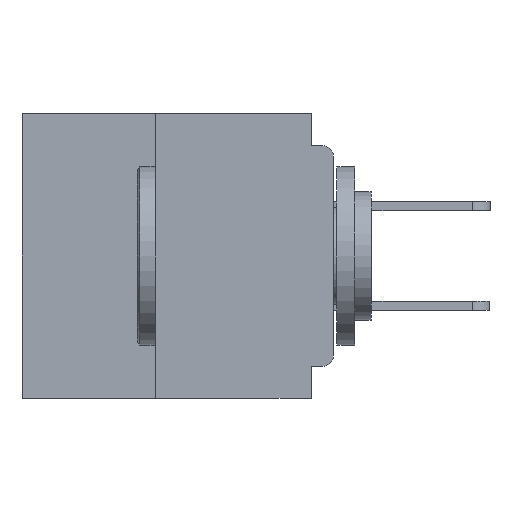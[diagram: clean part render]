
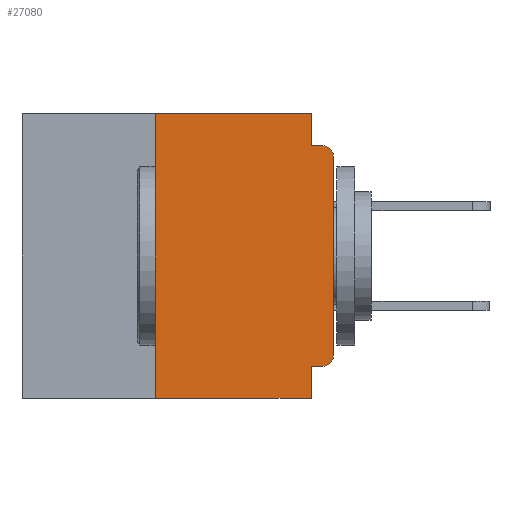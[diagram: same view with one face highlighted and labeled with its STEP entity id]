
A CAD part, left-side view. The second image highlights one B-rep face of the part: STEP entity #27080.
In plain terms, the highlighted planar face has unit normal (-1, 0, 0).
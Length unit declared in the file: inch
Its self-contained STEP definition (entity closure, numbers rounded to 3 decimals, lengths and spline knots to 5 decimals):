
#109 = EDGE_CURVE ( 'NONE', #25057, #23558, #26745, .T. ) ;
#2003 = CARTESIAN_POINT ( 'NONE',  ( 0., 0., -0.355 ) ) ;
#2442 = VERTEX_POINT ( 'NONE', #8196 ) ;
#2882 = DIRECTION ( 'NONE',  ( 0., 0., -1. ) ) ;
#3106 = LINE ( 'NONE', #30872, #19224 ) ;
#3540 = LINE ( 'NONE', #25709, #32822 ) ;
#3785 = CARTESIAN_POINT ( 'NONE',  ( 0., 0.031, 0. ) ) ;
#4992 = DIRECTION ( 'NONE',  ( 0., 1., 0. ) ) ;
#5091 = AXIS2_PLACEMENT_3D ( 'NONE', #8103, #27973, #10960 ) ;
#5327 = DIRECTION ( 'NONE',  ( 0., 0., 1. ) ) ;
#6253 = DIRECTION ( 'NONE',  ( 0., -1., 0. ) ) ;
#6867 = CARTESIAN_POINT ( 'NONE',  ( 0., 0.437, -0.4 ) ) ;
#7379 = DIRECTION ( 'NONE',  ( 0., -1., 0. ) ) ;
#8103 = CARTESIAN_POINT ( 'NONE',  ( 0., 0.015, -0.06 ) ) ;
#8196 = CARTESIAN_POINT ( 'NONE',  ( 0., 0., -0.34 ) ) ;
#8648 = CARTESIAN_POINT ( 'NONE',  ( 0., 0.25, 0. ) ) ;
#8846 = DIRECTION ( 'NONE',  ( -1., 0., 0. ) ) ;
#9642 = VERTEX_POINT ( 'NONE', #13099 ) ;
#9907 = VERTEX_POINT ( 'NONE', #28285 ) ;
#10299 = CARTESIAN_POINT ( 'NONE',  ( 0., 0.015, -0.045 ) ) ;
#10960 = DIRECTION ( 'NONE',  ( 0., 0., -1. ) ) ;
#11476 = VERTEX_POINT ( 'NONE', #10299 ) ;
#12678 = CARTESIAN_POINT ( 'NONE',  ( 0., 0.437, 0. ) ) ;
#13099 = CARTESIAN_POINT ( 'NONE',  ( 0., 0.031, -0.355 ) ) ;
#13114 = EDGE_LOOP ( 'NONE', ( #16177, #21460, #27855, #14474, #21971, #17206, #25708, #18022, #17857, #15685 ) ) ;
#13193 = EDGE_CURVE ( 'NONE', #27193, #2442, #21022, .T. ) ;
#13708 = EDGE_CURVE ( 'NONE', #25057, #18121, #3106, .T. ) ;
#13821 = EDGE_CURVE ( 'NONE', #9642, #23558, #36325, .T. ) ;
#14393 = LINE ( 'NONE', #2003, #35874 ) ;
#14474 = ORIENTED_EDGE ( 'NONE', *, *, #21185, .F. ) ;
#14938 = VECTOR ( 'NONE', #15388, 39.37008 ) ;
#15388 = DIRECTION ( 'NONE',  ( 0., 0., -1. ) ) ;
#15480 = LINE ( 'NONE', #35426, #22037 ) ;
#15609 = DIRECTION ( 'NONE',  ( 0., 0., -1. ) ) ;
#15685 = ORIENTED_EDGE ( 'NONE', *, *, #13193, .T. ) ;
#15722 = VECTOR ( 'NONE', #2882, 39.37008 ) ;
#16177 = ORIENTED_EDGE ( 'NONE', *, *, #30389, .T. ) ;
#16541 = CARTESIAN_POINT ( 'NONE',  ( 0., 0.031, -0.4 ) ) ;
#16759 = CIRCLE ( 'NONE', #5091, 0.015 ) ;
#17206 = ORIENTED_EDGE ( 'NONE', *, *, #13708, .F. ) ;
#17857 = ORIENTED_EDGE ( 'NONE', *, *, #22279, .F. ) ;
#18022 = ORIENTED_EDGE ( 'NONE', *, *, #13821, .F. ) ;
#18121 = VERTEX_POINT ( 'NONE', #8648 ) ;
#19160 = EDGE_CURVE ( 'NONE', #18121, #25252, #3540, .T. ) ;
#19224 = VECTOR ( 'NONE', #5327, 39.37008 ) ;
#19228 = VECTOR ( 'NONE', #6253, 39.37008 ) ;
#19791 = VERTEX_POINT ( 'NONE', #25541 ) ;
#21022 = CIRCLE ( 'NONE', #32841, 0.015 ) ;
#21185 = EDGE_CURVE ( 'NONE', #25252, #19791, #29005, .T. ) ;
#21460 = ORIENTED_EDGE ( 'NONE', *, *, #32525, .T. ) ;
#21971 = ORIENTED_EDGE ( 'NONE', *, *, #19160, .F. ) ;
#22037 = VECTOR ( 'NONE', #7379, 39.37008 ) ;
#22279 = EDGE_CURVE ( 'NONE', #27193, #9642, #14393, .T. ) ;
#22862 = CARTESIAN_POINT ( 'NONE',  ( 0., 0.031, -0.4 ) ) ;
#23393 = CARTESIAN_POINT ( 'NONE',  ( 0., 0., 0. ) ) ;
#23558 = VERTEX_POINT ( 'NONE', #16541 ) ;
#23712 = FACE_OUTER_BOUND ( 'NONE', #13114, .T. ) ;
#25057 = VERTEX_POINT ( 'NONE', #34355 ) ;
#25252 = VERTEX_POINT ( 'NONE', #35192 ) ;
#25541 = CARTESIAN_POINT ( 'NONE',  ( 0., 0.031, -0.045 ) ) ;
#25708 = ORIENTED_EDGE ( 'NONE', *, *, #109, .T. ) ;
#25709 = CARTESIAN_POINT ( 'NONE',  ( 0., 0.437, 0. ) ) ;
#25884 = CARTESIAN_POINT ( 'NONE',  ( 0., 0.015, -0.34 ) ) ;
#26271 = DIRECTION ( 'NONE',  ( 0., 0., 1. ) ) ;
#26745 = LINE ( 'NONE', #6867, #19228 ) ;
#27080 = ADVANCED_FACE ( 'NONE', ( #23712 ), #29628, .F. ) ;
#27193 = VERTEX_POINT ( 'NONE', #27280 ) ;
#27280 = CARTESIAN_POINT ( 'NONE',  ( 0., 0.015, -0.355 ) ) ;
#27554 = AXIS2_PLACEMENT_3D ( 'NONE', #12678, #32440, #15609 ) ;
#27855 = ORIENTED_EDGE ( 'NONE', *, *, #32421, .F. ) ;
#27973 = DIRECTION ( 'NONE',  ( -1., 0., 0. ) ) ;
#28285 = CARTESIAN_POINT ( 'NONE',  ( 0., 0., -0.06 ) ) ;
#28729 = DIRECTION ( 'NONE',  ( 0., 0., -1. ) ) ;
#29005 = LINE ( 'NONE', #3785, #14938 ) ;
#29287 = VECTOR ( 'NONE', #26271, 39.37008 ) ;
#29628 = PLANE ( 'NONE',  #27554 ) ;
#30389 = EDGE_CURVE ( 'NONE', #2442, #9907, #31022, .T. ) ;
#30872 = CARTESIAN_POINT ( 'NONE',  ( 0., 0.25, -0.4 ) ) ;
#31022 = LINE ( 'NONE', #23393, #29287 ) ;
#32421 = EDGE_CURVE ( 'NONE', #19791, #11476, #15480, .T. ) ;
#32440 = DIRECTION ( 'NONE',  ( 1., 0., 0. ) ) ;
#32525 = EDGE_CURVE ( 'NONE', #9907, #11476, #16759, .T. ) ;
#32822 = VECTOR ( 'NONE', #34155, 39.37008 ) ;
#32841 = AXIS2_PLACEMENT_3D ( 'NONE', #25884, #8846, #28729 ) ;
#34155 = DIRECTION ( 'NONE',  ( 0., -1., 0. ) ) ;
#34355 = CARTESIAN_POINT ( 'NONE',  ( 0., 0.25, -0.4 ) ) ;
#35192 = CARTESIAN_POINT ( 'NONE',  ( 0., 0.031, 0. ) ) ;
#35426 = CARTESIAN_POINT ( 'NONE',  ( 0., 0., -0.045 ) ) ;
#35874 = VECTOR ( 'NONE', #4992, 39.37008 ) ;
#36325 = LINE ( 'NONE', #22862, #15722 ) ;
